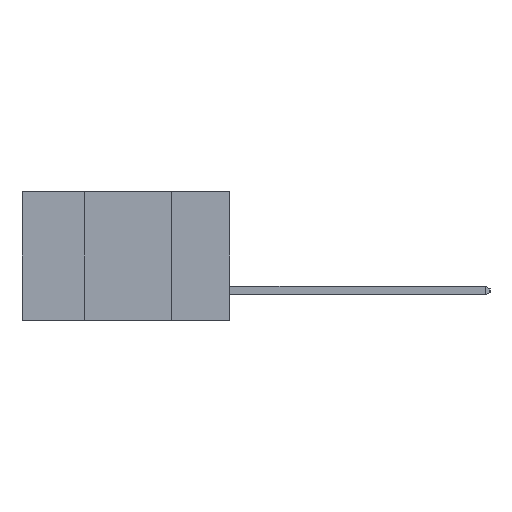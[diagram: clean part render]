
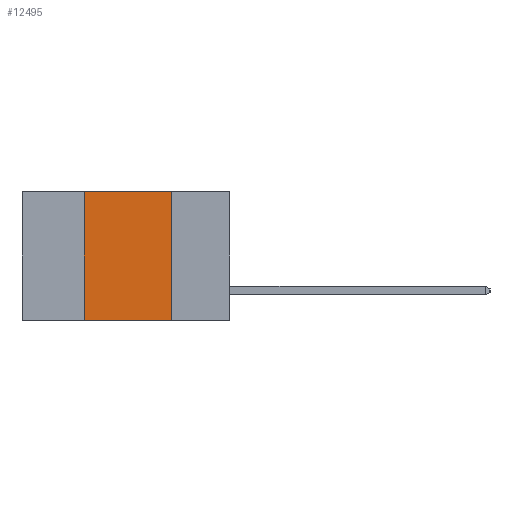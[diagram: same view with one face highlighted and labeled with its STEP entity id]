
A CAD part, left-side view. The second image highlights one B-rep face of the part: STEP entity #12495.
In plain terms, the highlighted planar face has unit normal (-1, 0, 0).
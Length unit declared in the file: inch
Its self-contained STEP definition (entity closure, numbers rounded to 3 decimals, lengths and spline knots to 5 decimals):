
#20 = VECTOR ( 'NONE', #17507, 39.37008 ) ;
#37 = VECTOR ( 'NONE', #2396, 39.37008 ) ;
#1976 = VERTEX_POINT ( 'NONE', #2681 ) ;
#2296 = CARTESIAN_POINT ( 'NONE',  ( 0., 0.17, -0.37 ) ) ;
#2396 = DIRECTION ( 'NONE',  ( 0., 0., -1. ) ) ;
#2681 = CARTESIAN_POINT ( 'NONE',  ( 0., 0.42, 0. ) ) ;
#3501 = PLANE ( 'NONE',  #12612 ) ;
#4784 = LINE ( 'NONE', #14298, #8766 ) ;
#4974 = LINE ( 'NONE', #15845, #20 ) ;
#5252 = DIRECTION ( 'NONE',  ( 1., 0., 0. ) ) ;
#5676 = EDGE_CURVE ( 'NONE', #11261, #12394, #13332, .T. ) ;
#6418 = FACE_OUTER_BOUND ( 'NONE', #8727, .T. ) ;
#8102 = EDGE_CURVE ( 'NONE', #9994, #1976, #9892, .T. ) ;
#8727 = EDGE_LOOP ( 'NONE', ( #13275, #18766, #13892, #14939 ) ) ;
#8766 = VECTOR ( 'NONE', #19233, 39.37008 ) ;
#8796 = DIRECTION ( 'NONE',  ( 0., 0., 1. ) ) ;
#9892 = LINE ( 'NONE', #18695, #18677 ) ;
#9994 = VERTEX_POINT ( 'NONE', #15624 ) ;
#10042 = CARTESIAN_POINT ( 'NONE',  ( 0., 0.17, -0.37 ) ) ;
#11261 = VERTEX_POINT ( 'NONE', #15505 ) ;
#12394 = VERTEX_POINT ( 'NONE', #10042 ) ;
#12495 = ADVANCED_FACE ( 'NONE', ( #6418 ), #3501, .F. ) ;
#12612 = AXIS2_PLACEMENT_3D ( 'NONE', #13469, #5252, #16892 ) ;
#13275 = ORIENTED_EDGE ( 'NONE', *, *, #5676, .F. ) ;
#13332 = LINE ( 'NONE', #2296, #37 ) ;
#13469 = CARTESIAN_POINT ( 'NONE',  ( 0., 0.6, 0. ) ) ;
#13892 = ORIENTED_EDGE ( 'NONE', *, *, #8102, .F. ) ;
#14298 = CARTESIAN_POINT ( 'NONE',  ( 0., 0.6, -0.37 ) ) ;
#14939 = ORIENTED_EDGE ( 'NONE', *, *, #21093, .T. ) ;
#15505 = CARTESIAN_POINT ( 'NONE',  ( 0., 0.17, 0. ) ) ;
#15624 = CARTESIAN_POINT ( 'NONE',  ( 0., 0.42, -0.37 ) ) ;
#15845 = CARTESIAN_POINT ( 'NONE',  ( 0., 0.6, 0. ) ) ;
#16655 = EDGE_CURVE ( 'NONE', #1976, #11261, #4974, .T. ) ;
#16892 = DIRECTION ( 'NONE',  ( 0., 0., -1. ) ) ;
#17507 = DIRECTION ( 'NONE',  ( 0., -1., 0. ) ) ;
#18677 = VECTOR ( 'NONE', #8796, 39.37008 ) ;
#18695 = CARTESIAN_POINT ( 'NONE',  ( 0., 0.42, -0.37 ) ) ;
#18766 = ORIENTED_EDGE ( 'NONE', *, *, #16655, .F. ) ;
#19233 = DIRECTION ( 'NONE',  ( 0., -1., 0. ) ) ;
#21093 = EDGE_CURVE ( 'NONE', #9994, #12394, #4784, .T. ) ;
